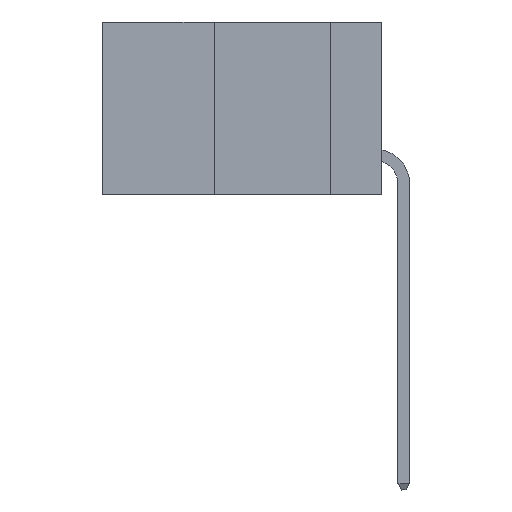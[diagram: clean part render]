
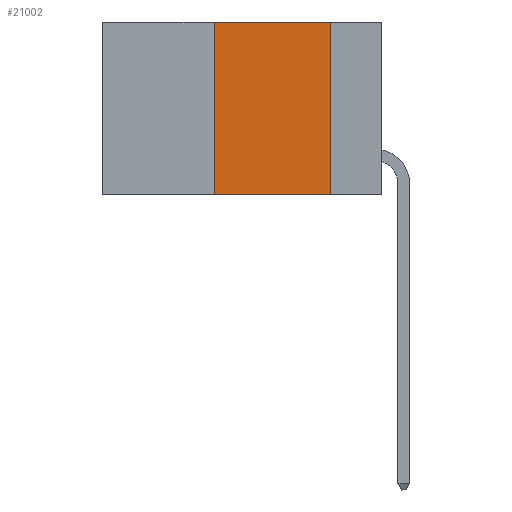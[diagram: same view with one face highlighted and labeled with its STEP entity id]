
A CAD part, left-side view. The second image highlights one B-rep face of the part: STEP entity #21002.
In plain terms, the highlighted planar face has unit normal (-1, 0, 0).
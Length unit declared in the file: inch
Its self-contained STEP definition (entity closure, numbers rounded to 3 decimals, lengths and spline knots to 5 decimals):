
#638 = VECTOR ( 'NONE', #4816, 39.37008 ) ;
#2819 = ORIENTED_EDGE ( 'NONE', *, *, #21321, .F. ) ;
#3165 = LINE ( 'NONE', #4982, #24361 ) ;
#3435 = AXIS2_PLACEMENT_3D ( 'NONE', #13999, #3443, #18218 ) ;
#3443 = DIRECTION ( 'NONE',  ( 1., 0., 0. ) ) ;
#4816 = DIRECTION ( 'NONE',  ( 0., -1., 0. ) ) ;
#4882 = CARTESIAN_POINT ( 'NONE',  ( 0., 0.11, 0. ) ) ;
#4982 = CARTESIAN_POINT ( 'NONE',  ( 0., 0.6, 0. ) ) ;
#5079 = DIRECTION ( 'NONE',  ( 0., -1., 0. ) ) ;
#5476 = PLANE ( 'NONE',  #3435 ) ;
#6305 = VERTEX_POINT ( 'NONE', #12381 ) ;
#7033 = CARTESIAN_POINT ( 'NONE',  ( 0., 0.6, -0.37 ) ) ;
#8899 = VERTEX_POINT ( 'NONE', #11010 ) ;
#10325 = EDGE_LOOP ( 'NONE', ( #2819, #10792, #20882, #11994 ) ) ;
#10792 = ORIENTED_EDGE ( 'NONE', *, *, #12276, .F. ) ;
#10799 = FACE_OUTER_BOUND ( 'NONE', #10325, .T. ) ;
#11010 = CARTESIAN_POINT ( 'NONE',  ( 0., 0.36, -0.37 ) ) ;
#11994 = ORIENTED_EDGE ( 'NONE', *, *, #26093, .T. ) ;
#12276 = EDGE_CURVE ( 'NONE', #16691, #24965, #3165, .T. ) ;
#12381 = CARTESIAN_POINT ( 'NONE',  ( 0., 0.11, -0.37 ) ) ;
#12444 = VECTOR ( 'NONE', #23686, 39.37008 ) ;
#13999 = CARTESIAN_POINT ( 'NONE',  ( 0., 0.6, 0. ) ) ;
#14021 = CARTESIAN_POINT ( 'NONE',  ( 0., 0.11, 0. ) ) ;
#14570 = CARTESIAN_POINT ( 'NONE',  ( 0., 0.36, 0. ) ) ;
#16691 = VERTEX_POINT ( 'NONE', #14570 ) ;
#17266 = LINE ( 'NONE', #22332, #17954 ) ;
#17954 = VECTOR ( 'NONE', #24022, 39.37008 ) ;
#18116 = LINE ( 'NONE', #4882, #12444 ) ;
#18218 = DIRECTION ( 'NONE',  ( 0., 0., -1. ) ) ;
#20882 = ORIENTED_EDGE ( 'NONE', *, *, #25676, .F. ) ;
#21002 = ADVANCED_FACE ( 'NONE', ( #10799 ), #5476, .F. ) ;
#21321 = EDGE_CURVE ( 'NONE', #24965, #6305, #18116, .T. ) ;
#21522 = LINE ( 'NONE', #7033, #638 ) ;
#22332 = CARTESIAN_POINT ( 'NONE',  ( 0., 0.36, 0. ) ) ;
#23686 = DIRECTION ( 'NONE',  ( 0., 0., -1. ) ) ;
#24022 = DIRECTION ( 'NONE',  ( 0., 0., 1. ) ) ;
#24361 = VECTOR ( 'NONE', #5079, 39.37008 ) ;
#24965 = VERTEX_POINT ( 'NONE', #14021 ) ;
#25676 = EDGE_CURVE ( 'NONE', #8899, #16691, #17266, .T. ) ;
#26093 = EDGE_CURVE ( 'NONE', #8899, #6305, #21522, .T. ) ;
